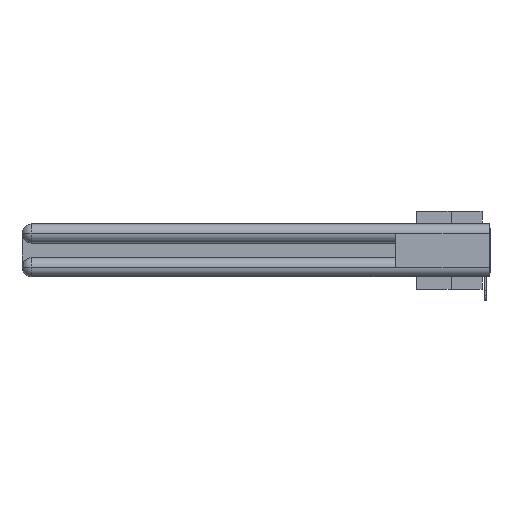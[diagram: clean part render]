
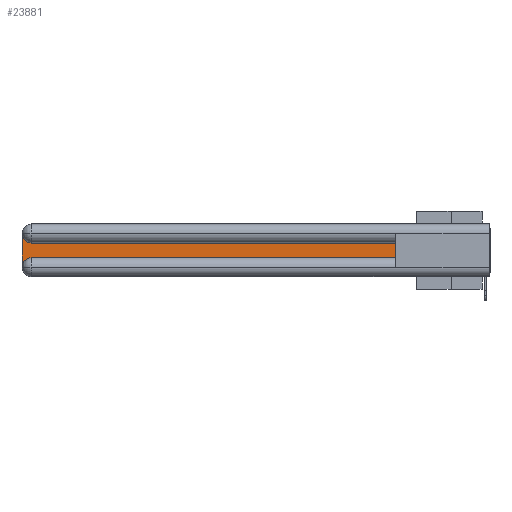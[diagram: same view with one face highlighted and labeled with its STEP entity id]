
A CAD part, left-side view. The second image highlights one B-rep face of the part: STEP entity #23881.
In plain terms, the highlighted planar face has unit normal (-1, 0, 0).
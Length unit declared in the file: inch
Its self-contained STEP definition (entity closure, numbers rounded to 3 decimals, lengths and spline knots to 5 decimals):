
#10 = CARTESIAN_POINT ( 'NONE',  ( 0.075, 3., -0.2775 ) ) ;
#236 = ORIENTED_EDGE ( 'NONE', *, *, #11013, .T. ) ;
#1267 = DIRECTION ( 'NONE',  ( 0., 0., -1. ) ) ;
#1572 = VECTOR ( 'NONE', #11159, 39.37008 ) ;
#2350 = EDGE_CURVE ( 'NONE', #24164, #27456, #21994, .T. ) ;
#2626 = LINE ( 'NONE', #10996, #1572 ) ;
#3205 = DIRECTION ( 'NONE',  ( 1., 0., 0. ) ) ;
#3344 = VECTOR ( 'NONE', #26640, 39.37008 ) ;
#5703 = CARTESIAN_POINT ( 'NONE',  ( 0.075, 0.6, -0.2175 ) ) ;
#6043 = LINE ( 'NONE', #5703, #11132 ) ;
#6979 = ORIENTED_EDGE ( 'NONE', *, *, #2350, .T. ) ;
#7988 = VERTEX_POINT ( 'NONE', #21384 ) ;
#8124 = VERTEX_POINT ( 'NONE', #9081 ) ;
#8771 = EDGE_CURVE ( 'NONE', #27456, #29248, #18345, .T. ) ;
#9081 = CARTESIAN_POINT ( 'NONE',  ( 0.075, 0.6, -0.2175 ) ) ;
#9199 = EDGE_CURVE ( 'NONE', #24482, #24164, #2626, .T. ) ;
#10767 = CARTESIAN_POINT ( 'NONE',  ( 0.075, 0.6, -0.2175 ) ) ;
#10996 = CARTESIAN_POINT ( 'NONE',  ( 0.075, 0.6, -0.1225 ) ) ;
#11013 = EDGE_CURVE ( 'NONE', #29248, #7988, #33718, .T. ) ;
#11132 = VECTOR ( 'NONE', #28765, 39.37008 ) ;
#11159 = DIRECTION ( 'NONE',  ( 0., 1., 0. ) ) ;
#11635 = FACE_OUTER_BOUND ( 'NONE', #19151, .T. ) ;
#12344 = VECTOR ( 'NONE', #16309, 39.37008 ) ;
#13409 = CARTESIAN_POINT ( 'NONE',  ( 0.075, 3., -0.2175 ) ) ;
#13659 = ORIENTED_EDGE ( 'NONE', *, *, #9199, .T. ) ;
#13814 = AXIS2_PLACEMENT_3D ( 'NONE', #16772, #14211, #1267 ) ;
#13927 = CARTESIAN_POINT ( 'NONE',  ( 0.075, 2.94, -0.2775 ) ) ;
#14211 = DIRECTION ( 'NONE',  ( 1., 0., 0. ) ) ;
#15476 = CARTESIAN_POINT ( 'NONE',  ( 0.075, 0.6, -0.1225 ) ) ;
#16233 = ORIENTED_EDGE ( 'NONE', *, *, #24100, .T. ) ;
#16309 = DIRECTION ( 'NONE',  ( 0., 0., -1. ) ) ;
#16772 = CARTESIAN_POINT ( 'NONE',  ( 0.075, 2.94, -0.0625 ) ) ;
#18345 = LINE ( 'NONE', #13409, #12344 ) ;
#18985 = AXIS2_PLACEMENT_3D ( 'NONE', #13927, #3205, #31870 ) ;
#19151 = EDGE_LOOP ( 'NONE', ( #13659, #6979, #22866, #236, #25052, #16233 ) ) ;
#19619 = DIRECTION ( 'NONE',  ( 0., 0., -1. ) ) ;
#21159 = LINE ( 'NONE', #10767, #3344 ) ;
#21384 = CARTESIAN_POINT ( 'NONE',  ( 0.075, 2.94, -0.2175 ) ) ;
#21994 = CIRCLE ( 'NONE', #13814, 0.06 ) ;
#22201 = PLANE ( 'NONE',  #28392 ) ;
#22363 = CARTESIAN_POINT ( 'NONE',  ( 0.075, 3., -0.1225 ) ) ;
#22866 = ORIENTED_EDGE ( 'NONE', *, *, #8771, .T. ) ;
#23881 = ADVANCED_FACE ( 'NONE', ( #11635 ), #22201, .F. ) ;
#24100 = EDGE_CURVE ( 'NONE', #8124, #24482, #21159, .T. ) ;
#24164 = VERTEX_POINT ( 'NONE', #27636 ) ;
#24482 = VERTEX_POINT ( 'NONE', #15476 ) ;
#25052 = ORIENTED_EDGE ( 'NONE', *, *, #28415, .T. ) ;
#26640 = DIRECTION ( 'NONE',  ( 0., 0., 1. ) ) ;
#27456 = VERTEX_POINT ( 'NONE', #31329 ) ;
#27636 = CARTESIAN_POINT ( 'NONE',  ( 0.075, 2.94, -0.1225 ) ) ;
#28392 = AXIS2_PLACEMENT_3D ( 'NONE', #22363, #32624, #19619 ) ;
#28415 = EDGE_CURVE ( 'NONE', #7988, #8124, #6043, .T. ) ;
#28765 = DIRECTION ( 'NONE',  ( 0., -1., 0. ) ) ;
#29248 = VERTEX_POINT ( 'NONE', #10 ) ;
#31329 = CARTESIAN_POINT ( 'NONE',  ( 0.075, 3., -0.0625 ) ) ;
#31870 = DIRECTION ( 'NONE',  ( 0., 0., -1. ) ) ;
#32624 = DIRECTION ( 'NONE',  ( 1., 0., 0. ) ) ;
#33718 = CIRCLE ( 'NONE', #18985, 0.06 ) ;
